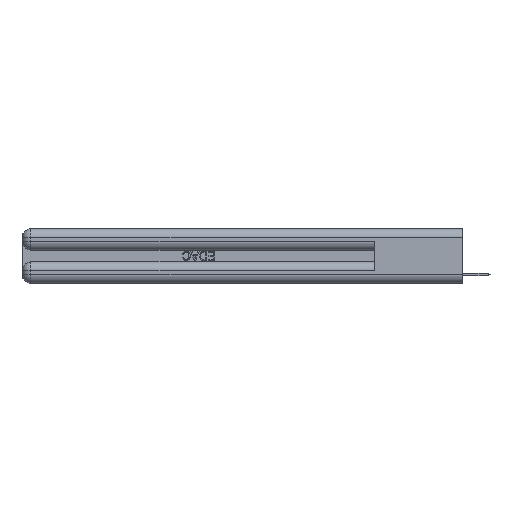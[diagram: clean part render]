
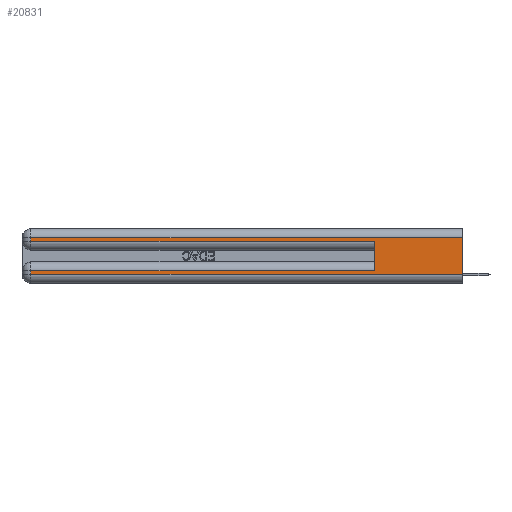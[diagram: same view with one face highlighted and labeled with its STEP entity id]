
A CAD part, left-side view. The second image highlights one B-rep face of the part: STEP entity #20831.
In plain terms, the highlighted planar face has unit normal (-1, 0, 0).
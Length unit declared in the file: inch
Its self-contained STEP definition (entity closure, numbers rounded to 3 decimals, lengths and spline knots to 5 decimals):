
#175 = VERTEX_POINT ( 'NONE', #20275 ) ;
#616 = VERTEX_POINT ( 'NONE', #18158 ) ;
#715 = ORIENTED_EDGE ( 'NONE', *, *, #9453, .F. ) ;
#4603 = CARTESIAN_POINT ( 'NONE',  ( 0., 0., 0.06 ) ) ;
#5224 = EDGE_CURVE ( 'NONE', #30409, #9548, #21556, .T. ) ;
#5622 = EDGE_CURVE ( 'NONE', #9548, #16511, #8025, .T. ) ;
#5778 = VECTOR ( 'NONE', #27054, 39.37008 ) ;
#5810 = EDGE_CURVE ( 'NONE', #175, #30409, #9510, .T. ) ;
#6967 = LINE ( 'NONE', #10519, #30542 ) ;
#6978 = CARTESIAN_POINT ( 'NONE',  ( 0., 0., 0.06 ) ) ;
#7893 = VECTOR ( 'NONE', #12688, 39.37008 ) ;
#8025 = LINE ( 'NONE', #6978, #23025 ) ;
#8167 = LINE ( 'NONE', #23532, #9676 ) ;
#8210 = EDGE_CURVE ( 'NONE', #24635, #20503, #20664, .T. ) ;
#8507 = ORIENTED_EDGE ( 'NONE', *, *, #16526, .F. ) ;
#9402 = CARTESIAN_POINT ( 'NONE',  ( 0., 2.94, 0.06 ) ) ;
#9453 = EDGE_CURVE ( 'NONE', #175, #616, #8167, .T. ) ;
#9510 = LINE ( 'NONE', #26944, #5778 ) ;
#9548 = VERTEX_POINT ( 'NONE', #9402 ) ;
#9676 = VECTOR ( 'NONE', #11423, 39.37008 ) ;
#10519 = CARTESIAN_POINT ( 'NONE',  ( 0., 2.94, 0.37 ) ) ;
#10706 = ORIENTED_EDGE ( 'NONE', *, *, #16645, .T. ) ;
#11423 = DIRECTION ( 'NONE',  ( 0., 0., 1. ) ) ;
#11565 = AXIS2_PLACEMENT_3D ( 'NONE', #25320, #18230, #27923 ) ;
#12688 = DIRECTION ( 'NONE',  ( 0., 1., 0. ) ) ;
#13393 = PLANE ( 'NONE',  #11565 ) ;
#14055 = VECTOR ( 'NONE', #28791, 39.37008 ) ;
#14684 = CARTESIAN_POINT ( 'NONE',  ( 0., 2.94, 0.31 ) ) ;
#14751 = CARTESIAN_POINT ( 'NONE',  ( 0., 0., 0.31 ) ) ;
#16511 = VERTEX_POINT ( 'NONE', #4603 ) ;
#16526 = EDGE_CURVE ( 'NONE', #24635, #16511, #21644, .T. ) ;
#16639 = DIRECTION ( 'NONE',  ( 0., -1., 0. ) ) ;
#16645 = EDGE_CURVE ( 'NONE', #20314, #616, #24691, .T. ) ;
#17350 = ORIENTED_EDGE ( 'NONE', *, *, #20358, .T. ) ;
#18158 = CARTESIAN_POINT ( 'NONE',  ( 0., 0.6, 0.285 ) ) ;
#18230 = DIRECTION ( 'NONE',  ( 1., 0., 0. ) ) ;
#19571 = DIRECTION ( 'NONE',  ( 0., -1., 0. ) ) ;
#19710 = EDGE_LOOP ( 'NONE', ( #8507, #22080, #17350, #10706, #715, #21300, #22755, #21716 ) ) ;
#20275 = CARTESIAN_POINT ( 'NONE',  ( 0., 0.6, 0.085 ) ) ;
#20314 = VERTEX_POINT ( 'NONE', #29556 ) ;
#20358 = EDGE_CURVE ( 'NONE', #20503, #20314, #6967, .T. ) ;
#20503 = VERTEX_POINT ( 'NONE', #14684 ) ;
#20664 = LINE ( 'NONE', #22324, #7893 ) ;
#20831 = ADVANCED_FACE ( 'NONE', ( #24175 ), #13393, .F. ) ;
#21300 = ORIENTED_EDGE ( 'NONE', *, *, #5810, .T. ) ;
#21556 = LINE ( 'NONE', #26382, #14055 ) ;
#21644 = LINE ( 'NONE', #26313, #30268 ) ;
#21679 = VECTOR ( 'NONE', #19571, 39.37008 ) ;
#21716 = ORIENTED_EDGE ( 'NONE', *, *, #5622, .T. ) ;
#22080 = ORIENTED_EDGE ( 'NONE', *, *, #8210, .T. ) ;
#22324 = CARTESIAN_POINT ( 'NONE',  ( 0., 0., 0.31 ) ) ;
#22755 = ORIENTED_EDGE ( 'NONE', *, *, #5224, .T. ) ;
#23025 = VECTOR ( 'NONE', #16639, 39.37008 ) ;
#23532 = CARTESIAN_POINT ( 'NONE',  ( 0., 0.6, 0.145 ) ) ;
#23913 = DIRECTION ( 'NONE',  ( 0., 0., -1. ) ) ;
#24175 = FACE_OUTER_BOUND ( 'NONE', #19710, .T. ) ;
#24635 = VERTEX_POINT ( 'NONE', #14751 ) ;
#24691 = LINE ( 'NONE', #29121, #21679 ) ;
#24954 = DIRECTION ( 'NONE',  ( 0., 0., -1. ) ) ;
#25320 = CARTESIAN_POINT ( 'NONE',  ( 0., 0., 0.37 ) ) ;
#26313 = CARTESIAN_POINT ( 'NONE',  ( 0., 0., 0.37 ) ) ;
#26382 = CARTESIAN_POINT ( 'NONE',  ( 0., 2.94, 0.37 ) ) ;
#26944 = CARTESIAN_POINT ( 'NONE',  ( 0., 0., 0.085 ) ) ;
#27054 = DIRECTION ( 'NONE',  ( 0., 1., 0. ) ) ;
#27923 = DIRECTION ( 'NONE',  ( 0., 0., -1. ) ) ;
#28791 = DIRECTION ( 'NONE',  ( 0., 0., -1. ) ) ;
#28979 = CARTESIAN_POINT ( 'NONE',  ( 0., 2.94, 0.085 ) ) ;
#29121 = CARTESIAN_POINT ( 'NONE',  ( 0., 0., 0.285 ) ) ;
#29556 = CARTESIAN_POINT ( 'NONE',  ( 0., 2.94, 0.285 ) ) ;
#30268 = VECTOR ( 'NONE', #23913, 39.37008 ) ;
#30409 = VERTEX_POINT ( 'NONE', #28979 ) ;
#30542 = VECTOR ( 'NONE', #24954, 39.37008 ) ;
